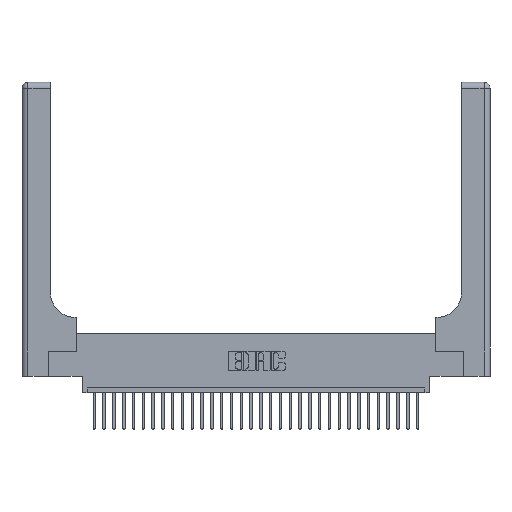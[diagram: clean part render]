
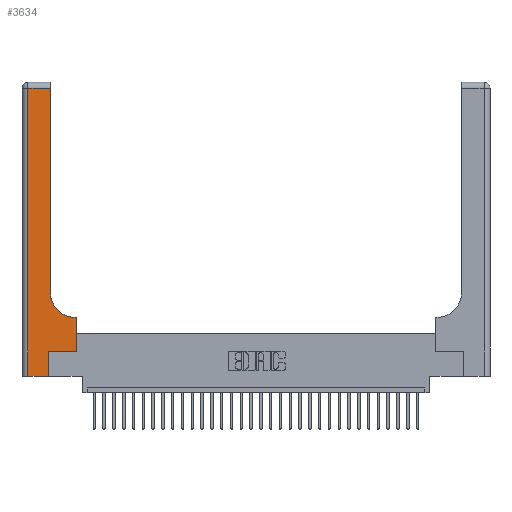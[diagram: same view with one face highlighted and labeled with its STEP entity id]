
A CAD part, top view. The second image highlights one B-rep face of the part: STEP entity #3634.
In plain terms, the highlighted planar face has unit normal (0, 0, 1).
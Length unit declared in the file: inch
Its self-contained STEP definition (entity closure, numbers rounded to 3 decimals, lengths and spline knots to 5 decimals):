
#25 = AXIS2_PLACEMENT_3D ( 'NONE', #1364, #13570, #26124 ) ;
#337 = VERTEX_POINT ( 'NONE', #3819 ) ;
#624 = EDGE_CURVE ( 'NONE', #6889, #16120, #10040, .T. ) ;
#1364 = CARTESIAN_POINT ( 'NONE',  ( 0.5415, 0.85, 0.37 ) ) ;
#1437 = EDGE_CURVE ( 'NONE', #6497, #14179, #12319, .T. ) ;
#2188 = LINE ( 'NONE', #23078, #28075 ) ;
#2680 = ORIENTED_EDGE ( 'NONE', *, *, #5314, .T. ) ;
#2707 = DIRECTION ( 'NONE',  ( -1., 0., 0. ) ) ;
#2788 = EDGE_CURVE ( 'NONE', #17001, #6889, #21560, .T. ) ;
#2984 = VECTOR ( 'NONE', #16933, 39.37008 ) ;
#3247 = CARTESIAN_POINT ( 'NONE',  ( 0.5585, 0.6, 0.37 ) ) ;
#3634 = ADVANCED_FACE ( 'NONE', ( #16848 ), #23982, .F. ) ;
#3734 = CARTESIAN_POINT ( 'NONE',  ( 0.06, 0., 0.37 ) ) ;
#3814 = DIRECTION ( 'NONE',  ( 0., 0., -1. ) ) ;
#3819 = CARTESIAN_POINT ( 'NONE',  ( 0.5415, 0.6, 0.37 ) ) ;
#4850 = VECTOR ( 'NONE', #25563, 39.37008 ) ;
#5314 = EDGE_CURVE ( 'NONE', #27421, #337, #26048, .T. ) ;
#5634 = DIRECTION ( 'NONE',  ( 0., 1., 0. ) ) ;
#6497 = VERTEX_POINT ( 'NONE', #28696 ) ;
#6889 = VERTEX_POINT ( 'NONE', #18603 ) ;
#7581 = CARTESIAN_POINT ( 'NONE',  ( 0., 2.94, 0.37 ) ) ;
#8431 = CARTESIAN_POINT ( 'NONE',  ( 0.06, 2.94, 0.37 ) ) ;
#8533 = ORIENTED_EDGE ( 'NONE', *, *, #624, .T. ) ;
#9673 = ORIENTED_EDGE ( 'NONE', *, *, #30786, .T. ) ;
#9993 = ORIENTED_EDGE ( 'NONE', *, *, #2788, .T. ) ;
#10040 = LINE ( 'NONE', #7581, #18199 ) ;
#11440 = LINE ( 'NONE', #16772, #12943 ) ;
#11903 = DIRECTION ( 'NONE',  ( 1., 0., 0. ) ) ;
#12077 = CARTESIAN_POINT ( 'NONE',  ( 0.06, 3., 0.37 ) ) ;
#12319 = LINE ( 'NONE', #31807, #2984 ) ;
#12943 = VECTOR ( 'NONE', #11903, 39.37008 ) ;
#13570 = DIRECTION ( 'NONE',  ( 0., 0., -1. ) ) ;
#13678 = CARTESIAN_POINT ( 'NONE',  ( 0.2915, 0.85, 0.37 ) ) ;
#13877 = CARTESIAN_POINT ( 'NONE',  ( 0., 3., 0.37 ) ) ;
#14039 = VECTOR ( 'NONE', #24634, 39.37008 ) ;
#14179 = VERTEX_POINT ( 'NONE', #31547 ) ;
#14652 = CARTESIAN_POINT ( 'NONE',  ( 0.2915, 0.6, 0.37 ) ) ;
#15410 = CARTESIAN_POINT ( 'NONE',  ( 0.2915, 3., 0.37 ) ) ;
#15884 = DIRECTION ( 'NONE',  ( 1., 0., 0. ) ) ;
#16120 = VERTEX_POINT ( 'NONE', #8431 ) ;
#16547 = EDGE_LOOP ( 'NONE', ( #9993, #8533, #26726, #29515, #17724, #18587, #19270, #2680, #9673 ) ) ;
#16772 = CARTESIAN_POINT ( 'NONE',  ( 0.269, 0.25, 0.37 ) ) ;
#16848 = FACE_OUTER_BOUND ( 'NONE', #16547, .T. ) ;
#16933 = DIRECTION ( 'NONE',  ( 0., 1., 0. ) ) ;
#17001 = VERTEX_POINT ( 'NONE', #13678 ) ;
#17154 = EDGE_CURVE ( 'NONE', #26932, #6497, #19197, .T. ) ;
#17724 = ORIENTED_EDGE ( 'NONE', *, *, #1437, .T. ) ;
#18199 = VECTOR ( 'NONE', #2707, 39.37008 ) ;
#18587 = ORIENTED_EDGE ( 'NONE', *, *, #20681, .T. ) ;
#18603 = CARTESIAN_POINT ( 'NONE',  ( 0.2915, 2.94, 0.37 ) ) ;
#18904 = CARTESIAN_POINT ( 'NONE',  ( 0.5585, 0.25, 0.37 ) ) ;
#18932 = EDGE_CURVE ( 'NONE', #16120, #26932, #19448, .T. ) ;
#19197 = LINE ( 'NONE', #23483, #21547 ) ;
#19270 = ORIENTED_EDGE ( 'NONE', *, *, #28096, .T. ) ;
#19448 = LINE ( 'NONE', #12077, #30991 ) ;
#20681 = EDGE_CURVE ( 'NONE', #14179, #29453, #11440, .T. ) ;
#21547 = VECTOR ( 'NONE', #15884, 39.37008 ) ;
#21560 = LINE ( 'NONE', #15410, #4850 ) ;
#23078 = CARTESIAN_POINT ( 'NONE',  ( 0.5585, 0.25, 0.37 ) ) ;
#23483 = CARTESIAN_POINT ( 'NONE',  ( 0., 0., 0.37 ) ) ;
#23982 = PLANE ( 'NONE',  #24934 ) ;
#24305 = DIRECTION ( 'NONE',  ( 0., -1., 0. ) ) ;
#24634 = DIRECTION ( 'NONE',  ( -1., 0., 0. ) ) ;
#24934 = AXIS2_PLACEMENT_3D ( 'NONE', #13877, #3814, #31161 ) ;
#25563 = DIRECTION ( 'NONE',  ( 0., 1., 0. ) ) ;
#26048 = LINE ( 'NONE', #14652, #14039 ) ;
#26124 = DIRECTION ( 'NONE',  ( 1., 0., 0. ) ) ;
#26726 = ORIENTED_EDGE ( 'NONE', *, *, #18932, .T. ) ;
#26932 = VERTEX_POINT ( 'NONE', #3734 ) ;
#27421 = VERTEX_POINT ( 'NONE', #3247 ) ;
#28075 = VECTOR ( 'NONE', #5634, 39.37008 ) ;
#28096 = EDGE_CURVE ( 'NONE', #29453, #27421, #2188, .T. ) ;
#28299 = CIRCLE ( 'NONE', #25, 0.25 ) ;
#28696 = CARTESIAN_POINT ( 'NONE',  ( 0.269, 0., 0.37 ) ) ;
#29453 = VERTEX_POINT ( 'NONE', #18904 ) ;
#29515 = ORIENTED_EDGE ( 'NONE', *, *, #17154, .T. ) ;
#30786 = EDGE_CURVE ( 'NONE', #337, #17001, #28299, .T. ) ;
#30991 = VECTOR ( 'NONE', #24305, 39.37008 ) ;
#31161 = DIRECTION ( 'NONE',  ( -1., 0., 0. ) ) ;
#31547 = CARTESIAN_POINT ( 'NONE',  ( 0.269, 0.25, 0.37 ) ) ;
#31807 = CARTESIAN_POINT ( 'NONE',  ( 0.269, 0., 0.37 ) ) ;
